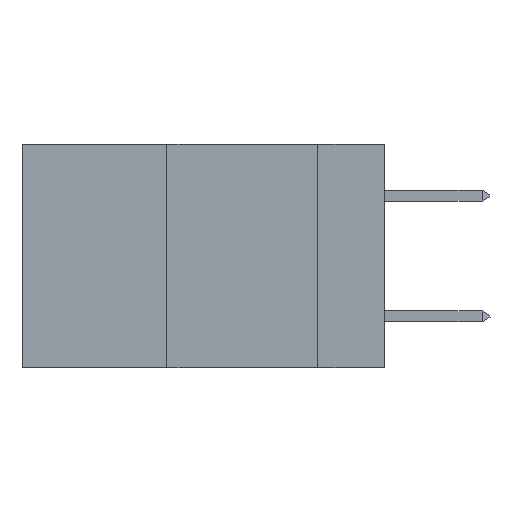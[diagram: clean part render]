
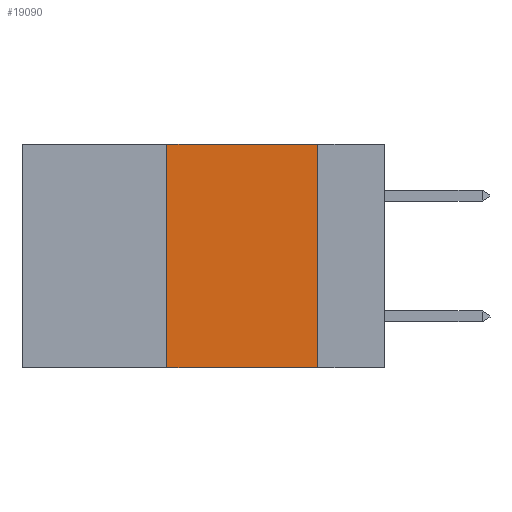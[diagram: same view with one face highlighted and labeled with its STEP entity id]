
A CAD part, left-side view. The second image highlights one B-rep face of the part: STEP entity #19090.
In plain terms, the highlighted planar face has unit normal (-1, 0, 0).
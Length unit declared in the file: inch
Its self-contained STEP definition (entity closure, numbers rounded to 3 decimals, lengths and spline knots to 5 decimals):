
#141 = VECTOR ( 'NONE', #13342, 39.37008 ) ;
#174 = DIRECTION ( 'NONE',  ( 0., 0., -1. ) ) ;
#3282 = CARTESIAN_POINT ( 'NONE',  ( 0., 0.36, -0.37 ) ) ;
#3456 = FACE_OUTER_BOUND ( 'NONE', #17454, .T. ) ;
#3932 = EDGE_CURVE ( 'NONE', #8604, #18723, #16354, .T. ) ;
#4001 = CARTESIAN_POINT ( 'NONE',  ( 0., 0.11, 0. ) ) ;
#4384 = LINE ( 'NONE', #8941, #11282 ) ;
#4406 = VERTEX_POINT ( 'NONE', #3282 ) ;
#5207 = EDGE_CURVE ( 'NONE', #18723, #12572, #9049, .T. ) ;
#5256 = CARTESIAN_POINT ( 'NONE',  ( 0., 0.6, 0. ) ) ;
#6115 = VECTOR ( 'NONE', #15987, 39.37008 ) ;
#6210 = CARTESIAN_POINT ( 'NONE',  ( 0., 0.11, 0. ) ) ;
#6607 = LINE ( 'NONE', #14433, #6115 ) ;
#7550 = CARTESIAN_POINT ( 'NONE',  ( 0., 0.11, -0.37 ) ) ;
#8048 = CARTESIAN_POINT ( 'NONE',  ( 0., 0.6, 0. ) ) ;
#8604 = VERTEX_POINT ( 'NONE', #16531 ) ;
#8941 = CARTESIAN_POINT ( 'NONE',  ( 0., 0.36, 0. ) ) ;
#9049 = LINE ( 'NONE', #4001, #141 ) ;
#9647 = DIRECTION ( 'NONE',  ( 1., 0., 0. ) ) ;
#10656 = EDGE_CURVE ( 'NONE', #4406, #8604, #4384, .T. ) ;
#10789 = ORIENTED_EDGE ( 'NONE', *, *, #3932, .F. ) ;
#11202 = PLANE ( 'NONE',  #17714 ) ;
#11282 = VECTOR ( 'NONE', #15157, 39.37008 ) ;
#11872 = ORIENTED_EDGE ( 'NONE', *, *, #10656, .F. ) ;
#12572 = VERTEX_POINT ( 'NONE', #7550 ) ;
#13342 = DIRECTION ( 'NONE',  ( 0., 0., -1. ) ) ;
#14433 = CARTESIAN_POINT ( 'NONE',  ( 0., 0.6, -0.37 ) ) ;
#15157 = DIRECTION ( 'NONE',  ( 0., 0., 1. ) ) ;
#15987 = DIRECTION ( 'NONE',  ( 0., -1., 0. ) ) ;
#16354 = LINE ( 'NONE', #5256, #19489 ) ;
#16531 = CARTESIAN_POINT ( 'NONE',  ( 0., 0.36, 0. ) ) ;
#17249 = ORIENTED_EDGE ( 'NONE', *, *, #19154, .T. ) ;
#17454 = EDGE_LOOP ( 'NONE', ( #19720, #10789, #11872, #17249 ) ) ;
#17703 = DIRECTION ( 'NONE',  ( 0., -1., 0. ) ) ;
#17714 = AXIS2_PLACEMENT_3D ( 'NONE', #8048, #9647, #174 ) ;
#18723 = VERTEX_POINT ( 'NONE', #6210 ) ;
#19090 = ADVANCED_FACE ( 'NONE', ( #3456 ), #11202, .F. ) ;
#19154 = EDGE_CURVE ( 'NONE', #4406, #12572, #6607, .T. ) ;
#19489 = VECTOR ( 'NONE', #17703, 39.37008 ) ;
#19720 = ORIENTED_EDGE ( 'NONE', *, *, #5207, .F. ) ;
